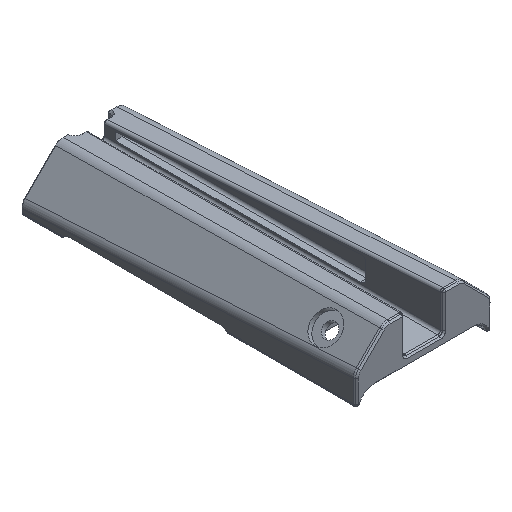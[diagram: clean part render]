
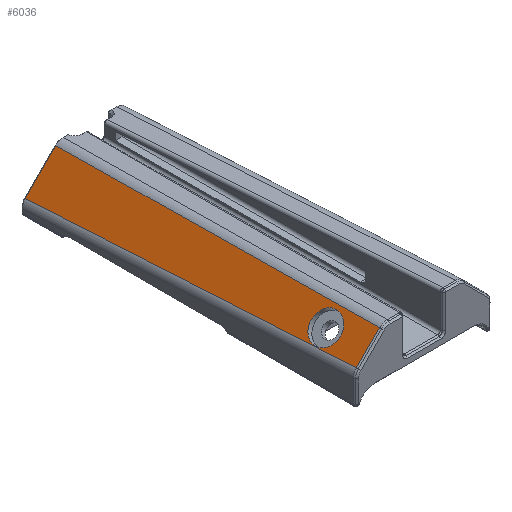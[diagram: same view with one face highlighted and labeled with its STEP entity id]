
A CAD part, isometric view. The second image highlights one B-rep face of the part: STEP entity #6036.
In plain terms, the highlighted planar face has unit normal (-0.707, 0.04, 0.706).
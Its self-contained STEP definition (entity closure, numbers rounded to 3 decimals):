
#62=FACE_BOUND('',#1034,.T.);
#87=B_SPLINE_CURVE_WITH_KNOTS('',3,(#8909,#8910,#8911,#8912),
 .UNSPECIFIED.,.F.,.F.,(4,4),(0.,0.001),.UNSPECIFIED.);
#89=B_SPLINE_CURVE_WITH_KNOTS('',3,(#8941,#8942,#8943,#8944),
 .UNSPECIFIED.,.F.,.F.,(4,4),(0.,0.001),
 .UNSPECIFIED.);
#134=B_SPLINE_CURVE_WITH_KNOTS('',3,(#9737,#9738,#9739,#9740),
 .UNSPECIFIED.,.F.,.F.,(4,4),(0.218,0.22),
 .UNSPECIFIED.);
#447=PLANE('',#6480);
#647=FACE_OUTER_BOUND('',#1033,.T.);
#1033=EDGE_LOOP('',(#4370,#4371,#4372,#4373,#4374,#4375,#4376));
#1034=EDGE_LOOP('',(#4377));
#1343=ELLIPSE('',#6412,2.802,2.8);
#1663=LINE('',#8923,#2091);
#1706=LINE('',#9734,#2134);
#1707=LINE('',#9742,#2135);
#1708=LINE('',#9743,#2136);
#2091=VECTOR('',#7110,10.);
#2134=VECTOR('',#7235,10.);
#2135=VECTOR('',#7238,10.);
#2136=VECTOR('',#7239,10.);
#2537=VERTEX_POINT('',#8778);
#2555=VERTEX_POINT('',#8865);
#2556=VERTEX_POINT('',#8905);
#2558=VERTEX_POINT('',#8908);
#2560=VERTEX_POINT('',#8920);
#2629=VERTEX_POINT('',#9729);
#2630=VERTEX_POINT('',#9736);
#2631=VERTEX_POINT('',#9741);
#3134=EDGE_CURVE('',#2537,#2537,#1343,.T.);
#3161=EDGE_CURVE('',#2558,#2556,#87,.T.);
#3165=EDGE_CURVE('',#2556,#2560,#1663,.T.);
#3167=EDGE_CURVE('',#2555,#2558,#89,.T.);
#3279=EDGE_CURVE('',#2560,#2629,#1706,.T.);
#3280=EDGE_CURVE('',#2629,#2630,#134,.T.);
#3281=EDGE_CURVE('',#2630,#2631,#1707,.T.);
#3282=EDGE_CURVE('',#2631,#2555,#1708,.T.);
#4370=ORIENTED_EDGE('',*,*,#3167,.T.);
#4371=ORIENTED_EDGE('',*,*,#3161,.T.);
#4372=ORIENTED_EDGE('',*,*,#3165,.T.);
#4373=ORIENTED_EDGE('',*,*,#3279,.T.);
#4374=ORIENTED_EDGE('',*,*,#3280,.T.);
#4375=ORIENTED_EDGE('',*,*,#3281,.T.);
#4376=ORIENTED_EDGE('',*,*,#3282,.T.);
#4377=ORIENTED_EDGE('',*,*,#3134,.F.);
#6036=ADVANCED_FACE('',(#647,#62),#447,.T.);
#6412=AXIS2_PLACEMENT_3D('',#8780,#7052,#7053);
#6480=AXIS2_PLACEMENT_3D('',#9735,#7236,#7237);
#7052=DIRECTION('center_axis',(-0.707,0.04,0.706));
#7053=DIRECTION('ref_axis',(0.026,0.999,-0.032));
#7110=DIRECTION('',(0.707,0.,0.707));
#7235=DIRECTION('',(0.022,0.999,-0.035));
#7236=DIRECTION('center_axis',(-0.707,0.04,0.706));
#7237=DIRECTION('ref_axis',(0.707,0.,0.707));
#7238=DIRECTION('',(-0.707,0.,-0.707));
#7239=DIRECTION('',(0.,-0.998,0.057));
#8778=CARTESIAN_POINT('',(-10.193,-0.028,7.825));
#8780=CARTESIAN_POINT('Origin',(-10.113,2.772,7.745));
#8865=CARTESIAN_POINT('',(-12.163,-4.991,6.137));
#8905=CARTESIAN_POINT('',(-12.147,-4.991,6.154));
#8908=CARTESIAN_POINT('',(-12.157,-4.991,6.143));
#8909=CARTESIAN_POINT('Ctrl Pts',(-12.157,-4.991,6.143));
#8910=CARTESIAN_POINT('Ctrl Pts',(-12.154,-4.991,6.147));
#8911=CARTESIAN_POINT('Ctrl Pts',(-12.15,-4.991,6.15));
#8912=CARTESIAN_POINT('Ctrl Pts',(-12.147,-4.991,6.154));
#8920=CARTESIAN_POINT('',(-7.791,-4.991,10.511));
#8923=CARTESIAN_POINT('',(-10.472,-4.991,7.83));
#8941=CARTESIAN_POINT('Ctrl Pts',(-12.163,-4.991,6.137));
#8942=CARTESIAN_POINT('Ctrl Pts',(-12.161,-4.991,6.139));
#8943=CARTESIAN_POINT('Ctrl Pts',(-12.159,-4.991,6.141));
#8944=CARTESIAN_POINT('Ctrl Pts',(-12.157,-4.991,6.143));
#9729=CARTESIAN_POINT('',(-6.415,57.139,8.342));
#9734=CARTESIAN_POINT('',(-7.008,30.376,9.276));
#9735=CARTESIAN_POINT('Origin',(-10.06,30.369,6.223));
#9736=CARTESIAN_POINT('',(-6.417,57.139,8.339));
#9737=CARTESIAN_POINT('Ctrl Pts',(-6.415,57.139,8.342));
#9738=CARTESIAN_POINT('Ctrl Pts',(-6.416,57.139,8.341));
#9739=CARTESIAN_POINT('Ctrl Pts',(-6.417,57.139,8.34));
#9740=CARTESIAN_POINT('Ctrl Pts',(-6.417,57.139,8.339));
#9741=CARTESIAN_POINT('',(-12.163,57.139,2.591));
#9742=CARTESIAN_POINT('',(-7.338,57.139,7.419));
#9743=CARTESIAN_POINT('',(-12.163,30.805,4.094));
